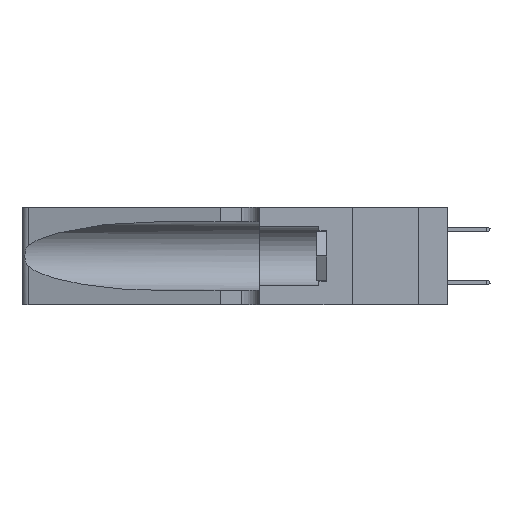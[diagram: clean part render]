
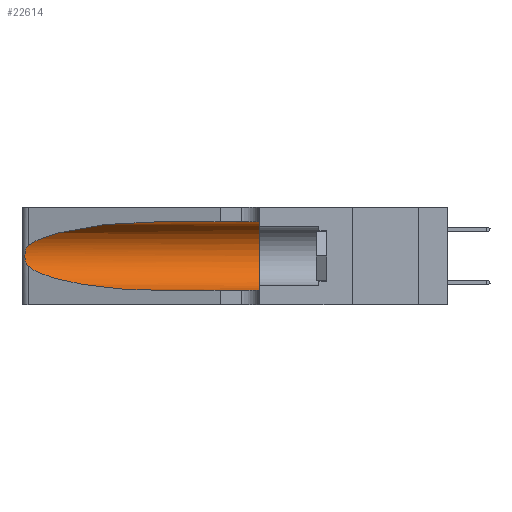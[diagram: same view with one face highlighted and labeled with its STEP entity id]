
A CAD part, left-side view. The second image highlights one B-rep face of the part: STEP entity #22614.
In plain terms, the highlighted cylindrical face has radius 3.308 mm (diameter 6.617 mm), a partial arc.
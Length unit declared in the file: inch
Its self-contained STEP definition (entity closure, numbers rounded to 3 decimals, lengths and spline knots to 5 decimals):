
#1743 = CARTESIAN_POINT ( 'NONE',  ( 0.2373, 1.15595, 0.08982 ) ) ;
#1826 = AXIS2_PLACEMENT_3D ( 'NONE', #31275, #38665, #45907 ) ;
#1987 = B_SPLINE_CURVE_WITH_KNOTS ( 'NONE', 3,
 ( #13745, #35782, #43151, #21195, #46877, #24892, #2757, #28562, #6481, #32235, #10206, #35948, #13904, #39625 ),
 .UNSPECIFIED., .F., .F.,
 ( 4, 2, 2, 2, 2, 2, 4 ),
 ( 0., 0.00027, 0.00053, 0.00107, 0.0016, 0.00187, 0.00214 ),
 .UNSPECIFIED. ) ;
#2617 = CARTESIAN_POINT ( 'NONE',  ( 0.1305, 0.72297, 0.31525 ) ) ;
#2757 = CARTESIAN_POINT ( 'NONE',  ( 0.26075, 1.23896, 0.19203 ) ) ;
#2833 = ORIENTED_EDGE ( 'NONE', *, *, #28626, .F. ) ;
#3701 = CARTESIAN_POINT ( 'NONE',  ( 0.1305, 0.72297, 0.05475 ) ) ;
#4192 = LINE ( 'NONE', #10628, #42187 ) ;
#6347 = CARTESIAN_POINT ( 'NONE',  ( 0.18966, 0.96281, 0.31525 ) ) ;
#6481 = CARTESIAN_POINT ( 'NONE',  ( 0.26017, 1.23833, 0.17102 ) ) ;
#8017 = ORIENTED_EDGE ( 'NONE', *, *, #11040, .F. ) ;
#9172 = CARTESIAN_POINT ( 'NONE',  ( 0.25487, 1.22718, 0.14631 ) ) ;
#10206 = CARTESIAN_POINT ( 'NONE',  ( 0.25789, 1.23486, 0.15765 ) ) ;
#10628 = CARTESIAN_POINT ( 'NONE',  ( 0.1305, 1.61858, 0.05475 ) ) ;
#11040 = EDGE_CURVE ( 'NONE', #44491, #12487, #24599, .T. ) ;
#11305 = EDGE_LOOP ( 'NONE', ( #34182, #47447, #19868, #33078, #8017, #2833 ) ) ;
#12487 = VERTEX_POINT ( 'NONE', #36462 ) ;
#13393 = CARTESIAN_POINT ( 'NONE',  ( 0.1305, 0.35, 0.185 ) ) ;
#13454 = LINE ( 'NONE', #17440, #30716 ) ;
#13745 = CARTESIAN_POINT ( 'NONE',  ( 0.25487, 1.22718, 0.22369 ) ) ;
#13768 = CARTESIAN_POINT ( 'NONE',  ( 0.25487, 1.22718, 0.22369 ) ) ;
#13904 = CARTESIAN_POINT ( 'NONE',  ( 0.25555, 1.22993, 0.14849 ) ) ;
#13908 = EDGE_CURVE ( 'NONE', #16265, #12487, #4192, .T. ) ;
#16265 = VERTEX_POINT ( 'NONE', #3701 ) ;
#16608 = CARTESIAN_POINT ( 'NONE',  ( 0.18966, 0.96281, 0.05475 ) ) ;
#17145 = DIRECTION ( 'NONE',  ( 0., 0., 1. ) ) ;
#17440 = CARTESIAN_POINT ( 'NONE',  ( 0.1305, 1.61858, 0.31525 ) ) ;
#19314 = VERTEX_POINT ( 'NONE', #44407 ) ;
#19868 = ORIENTED_EDGE ( 'NONE', *, *, #33855, .T. ) ;
#21195 = CARTESIAN_POINT ( 'NONE',  ( 0.25787, 1.23484, 0.2124 ) ) ;
#21310 = CARTESIAN_POINT ( 'NONE',  ( 0.1305, 0.35, 0.31525 ) ) ;
#22614 = ADVANCED_FACE ( 'NONE', ( #24586 ), #23400, .F. ) ;
#23317 = VERTEX_POINT ( 'NONE', #38611 ) ;
#23400 = CYLINDRICAL_SURFACE ( 'NONE', #1826, 0.13025 ) ;
#24354 = VERTEX_POINT ( 'NONE', #26676 ) ;
#24586 = FACE_OUTER_BOUND ( 'NONE', #11305, .T. ) ;
#24599 = CIRCLE ( 'NONE', #28129, 0.13025 ) ;
#24892 = CARTESIAN_POINT ( 'NONE',  ( 0.26018, 1.23835, 0.19895 ) ) ;
#26676 = CARTESIAN_POINT ( 'NONE',  ( 0.1305, 0.72297, 0.31525 ) ) ;
#28129 = AXIS2_PLACEMENT_3D ( 'NONE', #13393, #39134, #17145 ) ;
#28562 = CARTESIAN_POINT ( 'NONE',  ( 0.26075, 1.23896, 0.178 ) ) ;
#28626 = EDGE_CURVE ( 'NONE', #24354, #44491, #13454, .T. ) ;
#29877 = EDGE_CURVE ( 'NONE', #24354, #19314, #36263, .T. ) ;
#30716 = VECTOR ( 'NONE', #35910, 39.37008 ) ;
#31275 = CARTESIAN_POINT ( 'NONE',  ( 0.1305, 1.61858, 0.185 ) ) ;
#32235 = CARTESIAN_POINT ( 'NONE',  ( 0.25856, 1.23593, 0.16098 ) ) ;
#33078 = ORIENTED_EDGE ( 'NONE', *, *, #13908, .T. ) ;
#33388 = EDGE_CURVE ( 'NONE', #19314, #23317, #1987, .T. ) ;
#33855 = EDGE_CURVE ( 'NONE', #23317, #16265, #41216, .T. ) ;
#34182 = ORIENTED_EDGE ( 'NONE', *, *, #29877, .T. ) ;
#35782 = CARTESIAN_POINT ( 'NONE',  ( 0.25555, 1.22994, 0.2215 ) ) ;
#35808 = CARTESIAN_POINT ( 'NONE',  ( 0.2373, 1.15595, 0.28018 ) ) ;
#35910 = DIRECTION ( 'NONE',  ( 0., -1., 0. ) ) ;
#35948 = CARTESIAN_POINT ( 'NONE',  ( 0.25639, 1.23186, 0.15144 ) ) ;
#36263 =( BOUNDED_CURVE ( )  B_SPLINE_CURVE ( 3, ( #2617, #6347, #35808, #13768 ),
 .UNSPECIFIED., .F., .F. ) 
 B_SPLINE_CURVE_WITH_KNOTS ( ( 4, 4 ),
 ( 1.5708, 2.84003 ),
 .UNSPECIFIED. ) 
 CURVE ( )  GEOMETRIC_REPRESENTATION_ITEM ( )  RATIONAL_B_SPLINE_CURVE ( ( 1., 0.87, 0.87, 1. ) ) 
 REPRESENTATION_ITEM ( '' )  );
#36462 = CARTESIAN_POINT ( 'NONE',  ( 0.1305, 0.35, 0.05475 ) ) ;
#38611 = CARTESIAN_POINT ( 'NONE',  ( 0.25487, 1.22718, 0.14631 ) ) ;
#38665 = DIRECTION ( 'NONE',  ( 0., -1., 0. ) ) ;
#39134 = DIRECTION ( 'NONE',  ( 0., 1., 0. ) ) ;
#39625 = CARTESIAN_POINT ( 'NONE',  ( 0.25487, 1.22718, 0.14631 ) ) ;
#41216 =( BOUNDED_CURVE ( )  B_SPLINE_CURVE ( 3, ( #9172, #1743, #16608, #42286 ),
 .UNSPECIFIED., .F., .F. ) 
 B_SPLINE_CURVE_WITH_KNOTS ( ( 4, 4 ),
 ( 3.44316, 4.71239 ),
 .UNSPECIFIED. ) 
 CURVE ( )  GEOMETRIC_REPRESENTATION_ITEM ( )  RATIONAL_B_SPLINE_CURVE ( ( 1., 0.87, 0.87, 1. ) ) 
 REPRESENTATION_ITEM ( '' )  );
#42187 = VECTOR ( 'NONE', #43591, 39.37008 ) ;
#42286 = CARTESIAN_POINT ( 'NONE',  ( 0.1305, 0.72297, 0.05475 ) ) ;
#43151 = CARTESIAN_POINT ( 'NONE',  ( 0.25639, 1.23184, 0.21858 ) ) ;
#43591 = DIRECTION ( 'NONE',  ( 0., -1., 0. ) ) ;
#44407 = CARTESIAN_POINT ( 'NONE',  ( 0.25487, 1.22718, 0.22369 ) ) ;
#44491 = VERTEX_POINT ( 'NONE', #21310 ) ;
#45907 = DIRECTION ( 'NONE',  ( 0., 0., -1. ) ) ;
#46877 = CARTESIAN_POINT ( 'NONE',  ( 0.25854, 1.2359, 0.20912 ) ) ;
#47447 = ORIENTED_EDGE ( 'NONE', *, *, #33388, .T. ) ;
